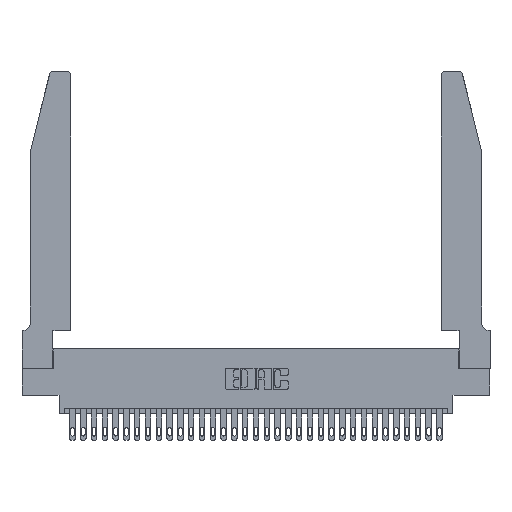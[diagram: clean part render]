
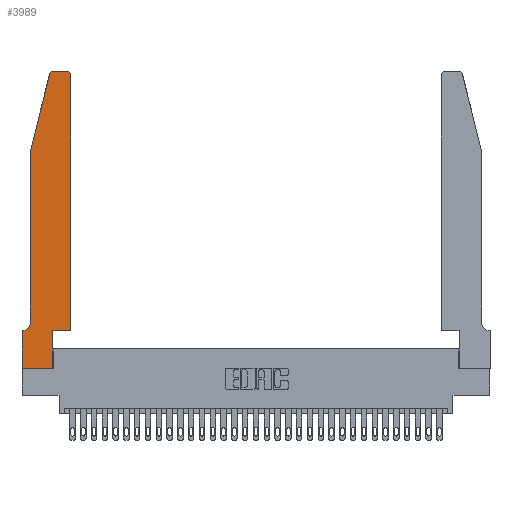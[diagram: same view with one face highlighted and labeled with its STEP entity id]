
A CAD part, top view. The second image highlights one B-rep face of the part: STEP entity #3989.
In plain terms, the highlighted planar face has unit normal (0, 0, 1).
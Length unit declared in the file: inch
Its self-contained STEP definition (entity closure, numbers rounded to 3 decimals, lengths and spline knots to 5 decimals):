
#175 = VECTOR ( 'NONE', #28785, 39.37008 ) ;
#403 = CARTESIAN_POINT ( 'NONE',  ( 0.0755, 2., 0.37 ) ) ;
#585 = VERTEX_POINT ( 'NONE', #20002 ) ;
#1497 = VERTEX_POINT ( 'NONE', #2893 ) ;
#2064 = CARTESIAN_POINT ( 'NONE',  ( 0.4505, 0.35, 0.37 ) ) ;
#2309 = LINE ( 'NONE', #14161, #6367 ) ;
#2396 = EDGE_CURVE ( 'NONE', #18912, #23582, #30683, .T. ) ;
#2659 = CIRCLE ( 'NONE', #30604, 0.03 ) ;
#2893 = CARTESIAN_POINT ( 'NONE',  ( 0.4505, 0.35, 0.37 ) ) ;
#2944 = EDGE_CURVE ( 'NONE', #2980, #26578, #24272, .T. ) ;
#2980 = VERTEX_POINT ( 'NONE', #24561 ) ;
#3238 = VERTEX_POINT ( 'NONE', #31519 ) ;
#3372 = PLANE ( 'NONE',  #22579 ) ;
#3482 = DIRECTION ( 'NONE',  ( 0., 1., 0. ) ) ;
#3989 = ADVANCED_FACE ( 'NONE', ( #32589 ), #3372, .T. ) ;
#4475 = ORIENTED_EDGE ( 'NONE', *, *, #4672, .T. ) ;
#4672 = EDGE_CURVE ( 'NONE', #23582, #1497, #5686, .T. ) ;
#5054 = VERTEX_POINT ( 'NONE', #9247 ) ;
#5158 = AXIS2_PLACEMENT_3D ( 'NONE', #32758, #22464, #27614 ) ;
#5187 = VERTEX_POINT ( 'NONE', #19875 ) ;
#5398 = VECTOR ( 'NONE', #26133, 39.37008 ) ;
#5686 = LINE ( 'NONE', #31835, #10494 ) ;
#6037 = ORIENTED_EDGE ( 'NONE', *, *, #7762, .T. ) ;
#6367 = VECTOR ( 'NONE', #29625, 39.37008 ) ;
#6527 = CARTESIAN_POINT ( 'NONE',  ( 0.2865, 0., 0.37 ) ) ;
#7622 = CARTESIAN_POINT ( 'NONE',  ( 0.0755, 2., 0.37 ) ) ;
#7762 = EDGE_CURVE ( 'NONE', #27067, #8607, #2659, .T. ) ;
#8016 = EDGE_CURVE ( 'NONE', #8607, #31117, #26999, .T. ) ;
#8310 = CIRCLE ( 'NONE', #25600, 0.07 ) ;
#8607 = VERTEX_POINT ( 'NONE', #15849 ) ;
#9247 = CARTESIAN_POINT ( 'NONE',  ( 0., 0.35, 0.37 ) ) ;
#9584 = EDGE_CURVE ( 'NONE', #585, #18912, #13842, .T. ) ;
#9612 = CIRCLE ( 'NONE', #5158, 0.03 ) ;
#10278 = EDGE_CURVE ( 'NONE', #26578, #5187, #32229, .T. ) ;
#10494 = VECTOR ( 'NONE', #21104, 39.37008 ) ;
#11132 = CARTESIAN_POINT ( 'NONE',  ( 0.2865, 0.35, 0.37 ) ) ;
#12259 = DIRECTION ( 'NONE',  ( 0., 0., -1. ) ) ;
#12508 = EDGE_CURVE ( 'NONE', #31117, #2980, #9612, .T. ) ;
#13025 = VECTOR ( 'NONE', #15337, 39.37008 ) ;
#13175 = CARTESIAN_POINT ( 'NONE',  ( 0.4505, 2.72, 0.37 ) ) ;
#13589 = DIRECTION ( 'NONE',  ( 1., 0., 0. ) ) ;
#13842 = LINE ( 'NONE', #15237, #13025 ) ;
#13844 = EDGE_CURVE ( 'NONE', #5187, #3238, #8310, .T. ) ;
#14002 = EDGE_LOOP ( 'NONE', ( #30432, #21223, #31679, #23579, #16001, #33096, #32862, #31171, #32339, #4475, #25733, #6037 ) ) ;
#14161 = CARTESIAN_POINT ( 'NONE',  ( 0.0755, 0.35, 0.37 ) ) ;
#15236 = CARTESIAN_POINT ( 'NONE',  ( 0., 0., 0.37 ) ) ;
#15237 = CARTESIAN_POINT ( 'NONE',  ( 0., 0., 0.37 ) ) ;
#15337 = DIRECTION ( 'NONE',  ( 1., 0., 0. ) ) ;
#15849 = CARTESIAN_POINT ( 'NONE',  ( 0.4205, 2.75, 0.37 ) ) ;
#15968 = CARTESIAN_POINT ( 'NONE',  ( 0.2865, 0.35, 0.37 ) ) ;
#16001 = ORIENTED_EDGE ( 'NONE', *, *, #13844, .T. ) ;
#16077 = VECTOR ( 'NONE', #20728, 39.37008 ) ;
#17356 = VECTOR ( 'NONE', #20243, 39.37008 ) ;
#17461 = EDGE_CURVE ( 'NONE', #1497, #27067, #25967, .T. ) ;
#18912 = VERTEX_POINT ( 'NONE', #6527 ) ;
#19495 = CARTESIAN_POINT ( 'NONE',  ( 0.4205, 2.72, 0.37 ) ) ;
#19786 = CARTESIAN_POINT ( 'NONE',  ( 0.284, 2.75, 0.37 ) ) ;
#19875 = CARTESIAN_POINT ( 'NONE',  ( 0.0755, 0.42, 0.37 ) ) ;
#20002 = CARTESIAN_POINT ( 'NONE',  ( 0., 0., 0.37 ) ) ;
#20243 = DIRECTION ( 'NONE',  ( 0., -1., 0. ) ) ;
#20728 = DIRECTION ( 'NONE',  ( -1., 0., 0. ) ) ;
#21104 = DIRECTION ( 'NONE',  ( 1., 0., 0. ) ) ;
#21223 = ORIENTED_EDGE ( 'NONE', *, *, #12508, .T. ) ;
#21753 = DIRECTION ( 'NONE',  ( 1., 0., 0. ) ) ;
#22464 = DIRECTION ( 'NONE',  ( 0., 0., 1. ) ) ;
#22579 = AXIS2_PLACEMENT_3D ( 'NONE', #26506, #26614, #13589 ) ;
#22598 = DIRECTION ( 'NONE',  ( -1., 0., 0. ) ) ;
#22737 = CARTESIAN_POINT ( 'NONE',  ( 0.0755, 2., 0.37 ) ) ;
#23563 = VECTOR ( 'NONE', #31876, 39.37008 ) ;
#23579 = ORIENTED_EDGE ( 'NONE', *, *, #10278, .T. ) ;
#23582 = VERTEX_POINT ( 'NONE', #15968 ) ;
#24272 = LINE ( 'NONE', #7622, #5398 ) ;
#24302 = LINE ( 'NONE', #15236, #175 ) ;
#24561 = CARTESIAN_POINT ( 'NONE',  ( 0.25487, 2.72718, 0.37 ) ) ;
#25524 = VECTOR ( 'NONE', #3482, 39.37008 ) ;
#25600 = AXIS2_PLACEMENT_3D ( 'NONE', #27203, #12259, #22598 ) ;
#25733 = ORIENTED_EDGE ( 'NONE', *, *, #17461, .T. ) ;
#25967 = LINE ( 'NONE', #2064, #23563 ) ;
#26133 = DIRECTION ( 'NONE',  ( -0.239, -0.971, 0. ) ) ;
#26506 = CARTESIAN_POINT ( 'NONE',  ( 0., 0.35, 0.37 ) ) ;
#26578 = VERTEX_POINT ( 'NONE', #403 ) ;
#26614 = DIRECTION ( 'NONE',  ( 0., 0., 1. ) ) ;
#26999 = LINE ( 'NONE', #30788, #16077 ) ;
#27067 = VERTEX_POINT ( 'NONE', #13175 ) ;
#27203 = CARTESIAN_POINT ( 'NONE',  ( 0.0055, 0.42, 0.37 ) ) ;
#27614 = DIRECTION ( 'NONE',  ( 1., 0., 0. ) ) ;
#28157 = EDGE_CURVE ( 'NONE', #5054, #585, #24302, .T. ) ;
#28785 = DIRECTION ( 'NONE',  ( 0., -1., 0. ) ) ;
#29625 = DIRECTION ( 'NONE',  ( -1., 0., 0. ) ) ;
#29661 = EDGE_CURVE ( 'NONE', #3238, #5054, #2309, .T. ) ;
#29688 = DIRECTION ( 'NONE',  ( 0., 0., 1. ) ) ;
#30432 = ORIENTED_EDGE ( 'NONE', *, *, #8016, .T. ) ;
#30604 = AXIS2_PLACEMENT_3D ( 'NONE', #19495, #29688, #21753 ) ;
#30683 = LINE ( 'NONE', #11132, #25524 ) ;
#30788 = CARTESIAN_POINT ( 'NONE',  ( 0.2605, 2.75, 0.37 ) ) ;
#31117 = VERTEX_POINT ( 'NONE', #19786 ) ;
#31171 = ORIENTED_EDGE ( 'NONE', *, *, #9584, .T. ) ;
#31519 = CARTESIAN_POINT ( 'NONE',  ( 0.0055, 0.35, 0.37 ) ) ;
#31679 = ORIENTED_EDGE ( 'NONE', *, *, #2944, .T. ) ;
#31835 = CARTESIAN_POINT ( 'NONE',  ( 0.4505, 0.35, 0.37 ) ) ;
#31876 = DIRECTION ( 'NONE',  ( 0., 1., 0. ) ) ;
#32229 = LINE ( 'NONE', #22737, #17356 ) ;
#32339 = ORIENTED_EDGE ( 'NONE', *, *, #2396, .T. ) ;
#32589 = FACE_OUTER_BOUND ( 'NONE', #14002, .T. ) ;
#32758 = CARTESIAN_POINT ( 'NONE',  ( 0.284, 2.72, 0.37 ) ) ;
#32862 = ORIENTED_EDGE ( 'NONE', *, *, #28157, .T. ) ;
#33096 = ORIENTED_EDGE ( 'NONE', *, *, #29661, .T. ) ;
